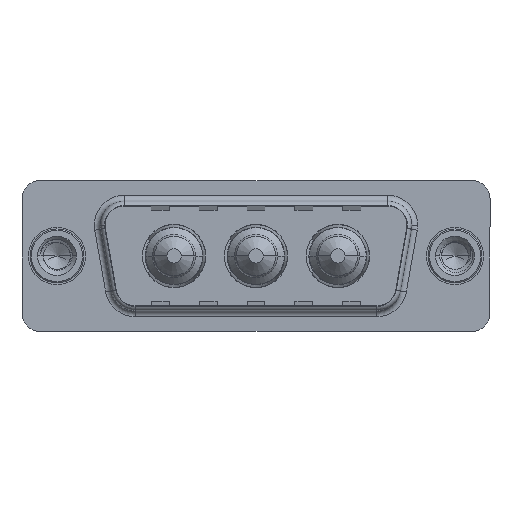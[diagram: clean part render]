
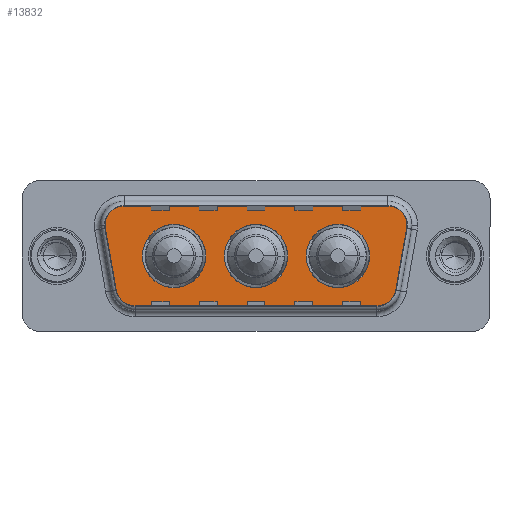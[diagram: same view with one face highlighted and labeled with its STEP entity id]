
A CAD part, top view. The second image highlights one B-rep face of the part: STEP entity #13832.
In plain terms, the highlighted planar face has unit normal (0, 0, 1).
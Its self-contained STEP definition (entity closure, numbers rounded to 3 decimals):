
#61 = DIRECTION ( 'NONE',  ( 0., 0., 1. ) ) ;
#78 = AXIS2_PLACEMENT_3D ( 'NONE', #301, #9163, #1596 ) ;
#163 = EDGE_CURVE ( 'NONE', #9623, #9041, #13083, .T. ) ;
#291 = CIRCLE ( 'NONE', #7058, 2.65 ) ;
#301 = CARTESIAN_POINT ( 'NONE',  ( 6.434, -2.9, 0. ) ) ;
#304 = CARTESIAN_POINT ( 'NONE',  ( 26.866, -2.9, 0. ) ) ;
#387 = EDGE_CURVE ( 'NONE', #11816, #12930, #13210, .T. ) ;
#466 = DIRECTION ( 'NONE',  ( 0., 0., 1. ) ) ;
#569 = VERTEX_POINT ( 'NONE', #11325 ) ;
#781 = EDGE_CURVE ( 'NONE', #16310, #8497, #2176, .T. ) ;
#783 = CIRCLE ( 'NONE', #78, 2. ) ;
#862 = ORIENTED_EDGE ( 'NONE', *, *, #2254, .F. ) ;
#960 = EDGE_LOOP ( 'NONE', ( #14982, #11648 ) ) ;
#1304 = ORIENTED_EDGE ( 'NONE', *, *, #15572, .T. ) ;
#1589 = AXIS2_PLACEMENT_3D ( 'NONE', #7036, #9707, #8698 ) ;
#1596 = DIRECTION ( 'NONE',  ( -1., 0., 0. ) ) ;
#1604 = CIRCLE ( 'NONE', #14845, 2.65 ) ;
#1713 = DIRECTION ( 'NONE',  ( 1., 0., 0. ) ) ;
#2176 = CIRCLE ( 'NONE', #6014, 2. ) ;
#2254 = EDGE_CURVE ( 'NONE', #11732, #569, #14954, .T. ) ;
#2324 = CIRCLE ( 'NONE', #15003, 2. ) ;
#2423 = EDGE_CURVE ( 'NONE', #12930, #9623, #12947, .T. ) ;
#2618 = DIRECTION ( 'NONE',  ( 1., 0., 0. ) ) ;
#2625 = CARTESIAN_POINT ( 'NONE',  ( 29.859, 2.553, 0. ) ) ;
#2858 = CARTESIAN_POINT ( 'NONE',  ( 5.411, 4.9, 0. ) ) ;
#2860 = EDGE_CURVE ( 'NONE', #15848, #16310, #4694, .T. ) ;
#2887 = EDGE_CURVE ( 'NONE', #12675, #8812, #14366, .T. ) ;
#2980 = DIRECTION ( 'NONE',  ( 0., 0., 1. ) ) ;
#3108 = ORIENTED_EDGE ( 'NONE', *, *, #163, .T. ) ;
#3257 = EDGE_CURVE ( 'NONE', #569, #11732, #13745, .T. ) ;
#3400 = CARTESIAN_POINT ( 'NONE',  ( 9.8, 0., 0. ) ) ;
#3410 = CARTESIAN_POINT ( 'NONE',  ( 3.441, 2.553, 0. ) ) ;
#3514 = AXIS2_PLACEMENT_3D ( 'NONE', #6368, #4730, #14247 ) ;
#3944 = ORIENTED_EDGE ( 'NONE', *, *, #781, .T. ) ;
#3976 = DIRECTION ( 'NONE',  ( 1., 0., 0. ) ) ;
#4053 = EDGE_CURVE ( 'NONE', #8812, #12675, #10983, .T. ) ;
#4225 = DIRECTION ( 'NONE',  ( -1., 0., 0. ) ) ;
#4395 = CARTESIAN_POINT ( 'NONE',  ( 3.441, 2.553, 0. ) ) ;
#4661 = DIRECTION ( 'NONE',  ( 1., 0., 0. ) ) ;
#4681 = ORIENTED_EDGE ( 'NONE', *, *, #2887, .F. ) ;
#4694 = LINE ( 'NONE', #5410, #11018 ) ;
#4699 = CARTESIAN_POINT ( 'NONE',  ( 26.866, -2.9, 0. ) ) ;
#4730 = DIRECTION ( 'NONE',  ( 0., 0., 1. ) ) ;
#4750 = CARTESIAN_POINT ( 'NONE',  ( 14., 0., 0. ) ) ;
#4872 = ORIENTED_EDGE ( 'NONE', *, *, #9179, .T. ) ;
#4978 = FACE_OUTER_BOUND ( 'NONE', #7651, .T. ) ;
#5063 = DIRECTION ( 'NONE',  ( -1., 0., 0. ) ) ;
#5396 = DIRECTION ( 'NONE',  ( 1., 0., 0. ) ) ;
#5410 = CARTESIAN_POINT ( 'NONE',  ( 6.434, -4.9, 0. ) ) ;
#5851 = CARTESIAN_POINT ( 'NONE',  ( 26.866, -4.9, 0. ) ) ;
#6014 = AXIS2_PLACEMENT_3D ( 'NONE', #4699, #9716, #1713 ) ;
#6122 = DIRECTION ( 'NONE',  ( 0.174, 0.985, 0. ) ) ;
#6132 = EDGE_CURVE ( 'NONE', #15723, #11286, #1604, .T. ) ;
#6368 = CARTESIAN_POINT ( 'NONE',  ( 23.5, 0., 0. ) ) ;
#6400 = CARTESIAN_POINT ( 'NONE',  ( 23.5, 0., 0. ) ) ;
#6404 = CARTESIAN_POINT ( 'NONE',  ( 27.889, 4.9, 0. ) ) ;
#6472 = CARTESIAN_POINT ( 'NONE',  ( 27.889, 2.9, 0. ) ) ;
#7036 = CARTESIAN_POINT ( 'NONE',  ( 5.411, 2.9, 0. ) ) ;
#7058 = AXIS2_PLACEMENT_3D ( 'NONE', #8048, #466, #9312 ) ;
#7291 = EDGE_LOOP ( 'NONE', ( #11979, #4681 ) ) ;
#7331 = AXIS2_PLACEMENT_3D ( 'NONE', #6400, #61, #2618 ) ;
#7557 = FACE_BOUND ( 'NONE', #7291, .T. ) ;
#7565 = CARTESIAN_POINT ( 'NONE',  ( 5.411, 4.9, 0. ) ) ;
#7587 = CARTESIAN_POINT ( 'NONE',  ( 6.434, -4.9, 0. ) ) ;
#7651 = EDGE_LOOP ( 'NONE', ( #3944, #4872, #14898, #15714, #13138, #3108, #11082, #1304, #13978 ) ) ;
#7766 = DIRECTION ( 'NONE',  ( -1., 0., 0. ) ) ;
#8017 = AXIS2_PLACEMENT_3D ( 'NONE', #304, #12959, #5396 ) ;
#8048 = CARTESIAN_POINT ( 'NONE',  ( 9.8, 0., 0. ) ) ;
#8497 = VERTEX_POINT ( 'NONE', #10308 ) ;
#8698 = DIRECTION ( 'NONE',  ( 1., 0., 0. ) ) ;
#8812 = VERTEX_POINT ( 'NONE', #12828 ) ;
#9041 = VERTEX_POINT ( 'NONE', #3410 ) ;
#9163 = DIRECTION ( 'NONE',  ( 0., 0., 1. ) ) ;
#9179 = EDGE_CURVE ( 'NONE', #8497, #12902, #10656, .T. ) ;
#9204 = VECTOR ( 'NONE', #5063, 1000. ) ;
#9312 = DIRECTION ( 'NONE',  ( 1., 0., 0. ) ) ;
#9623 = VERTEX_POINT ( 'NONE', #2858 ) ;
#9707 = DIRECTION ( 'NONE',  ( 0., 0., 1. ) ) ;
#9716 = DIRECTION ( 'NONE',  ( 0., 0., 1. ) ) ;
#9951 = EDGE_LOOP ( 'NONE', ( #15426, #862 ) ) ;
#10010 = CARTESIAN_POINT ( 'NONE',  ( 29.889, 2.9, 0. ) ) ;
#10082 = CARTESIAN_POINT ( 'NONE',  ( 12.45, 0., 0. ) ) ;
#10250 = DIRECTION ( 'NONE',  ( 1., 0., 0. ) ) ;
#10308 = CARTESIAN_POINT ( 'NONE',  ( 28.836, -3.247, 0. ) ) ;
#10428 = PLANE ( 'NONE',  #8017 ) ;
#10656 = LINE ( 'NONE', #16272, #13998 ) ;
#10679 = VECTOR ( 'NONE', #13199, 1000. ) ;
#10929 = FACE_BOUND ( 'NONE', #9951, .T. ) ;
#10983 = CIRCLE ( 'NONE', #15707, 2.65 ) ;
#11018 = VECTOR ( 'NONE', #10250, 1000. ) ;
#11082 = ORIENTED_EDGE ( 'NONE', *, *, #15251, .T. ) ;
#11087 = LINE ( 'NONE', #4395, #10679 ) ;
#11286 = VERTEX_POINT ( 'NONE', #10082 ) ;
#11325 = CARTESIAN_POINT ( 'NONE',  ( 26.15, 0., 0. ) ) ;
#11386 = DIRECTION ( 'NONE',  ( 0., 0., 1. ) ) ;
#11648 = ORIENTED_EDGE ( 'NONE', *, *, #6132, .F. ) ;
#11732 = VERTEX_POINT ( 'NONE', #13401 ) ;
#11816 = VERTEX_POINT ( 'NONE', #10010 ) ;
#11872 = EDGE_CURVE ( 'NONE', #12902, #11816, #2324, .T. ) ;
#11979 = ORIENTED_EDGE ( 'NONE', *, *, #4053, .F. ) ;
#12032 = EDGE_CURVE ( 'NONE', #11286, #15723, #291, .T. ) ;
#12219 = DIRECTION ( 'NONE',  ( 0., 0., 1. ) ) ;
#12675 = VERTEX_POINT ( 'NONE', #4750 ) ;
#12828 = CARTESIAN_POINT ( 'NONE',  ( 19.3, 0., 0. ) ) ;
#12902 = VERTEX_POINT ( 'NONE', #2625 ) ;
#12930 = VERTEX_POINT ( 'NONE', #6404 ) ;
#12947 = LINE ( 'NONE', #7565, #9204 ) ;
#12959 = DIRECTION ( 'NONE',  ( 0., 0., 1. ) ) ;
#13016 = AXIS2_PLACEMENT_3D ( 'NONE', #13059, #2980, #3976 ) ;
#13059 = CARTESIAN_POINT ( 'NONE',  ( 16.65, 0., 0. ) ) ;
#13083 = CIRCLE ( 'NONE', #1589, 2. ) ;
#13138 = ORIENTED_EDGE ( 'NONE', *, *, #2423, .T. ) ;
#13199 = DIRECTION ( 'NONE',  ( 0.174, -0.985, 0. ) ) ;
#13210 = CIRCLE ( 'NONE', #16015, 2. ) ;
#13278 = DIRECTION ( 'NONE',  ( 0., 0., 1. ) ) ;
#13375 = VERTEX_POINT ( 'NONE', #14599 ) ;
#13401 = CARTESIAN_POINT ( 'NONE',  ( 20.85, 0., 0. ) ) ;
#13699 = CARTESIAN_POINT ( 'NONE',  ( 16.65, 0., 0. ) ) ;
#13745 = CIRCLE ( 'NONE', #7331, 2.65 ) ;
#13832 = ADVANCED_FACE ( 'NONE', ( #7557, #10929, #13861, #4978 ), #10428, .T. ) ;
#13861 = FACE_BOUND ( 'NONE', #960, .T. ) ;
#13978 = ORIENTED_EDGE ( 'NONE', *, *, #2860, .T. ) ;
#13998 = VECTOR ( 'NONE', #6122, 1000. ) ;
#14247 = DIRECTION ( 'NONE',  ( 1., 0., 0. ) ) ;
#14366 = CIRCLE ( 'NONE', #13016, 2.65 ) ;
#14404 = CARTESIAN_POINT ( 'NONE',  ( 27.889, 2.9, 0. ) ) ;
#14599 = CARTESIAN_POINT ( 'NONE',  ( 4.464, -3.247, 0. ) ) ;
#14845 = AXIS2_PLACEMENT_3D ( 'NONE', #3400, #12219, #4661 ) ;
#14898 = ORIENTED_EDGE ( 'NONE', *, *, #11872, .T. ) ;
#14954 = CIRCLE ( 'NONE', #3514, 2.65 ) ;
#14982 = ORIENTED_EDGE ( 'NONE', *, *, #12032, .F. ) ;
#15003 = AXIS2_PLACEMENT_3D ( 'NONE', #6472, #15335, #7766 ) ;
#15251 = EDGE_CURVE ( 'NONE', #9041, #13375, #11087, .T. ) ;
#15335 = DIRECTION ( 'NONE',  ( 0., 0., 1. ) ) ;
#15426 = ORIENTED_EDGE ( 'NONE', *, *, #3257, .F. ) ;
#15572 = EDGE_CURVE ( 'NONE', #13375, #15848, #783, .T. ) ;
#15707 = AXIS2_PLACEMENT_3D ( 'NONE', #13699, #13278, #15776 ) ;
#15714 = ORIENTED_EDGE ( 'NONE', *, *, #387, .T. ) ;
#15723 = VERTEX_POINT ( 'NONE', #15861 ) ;
#15776 = DIRECTION ( 'NONE',  ( 1., 0., 0. ) ) ;
#15848 = VERTEX_POINT ( 'NONE', #7587 ) ;
#15861 = CARTESIAN_POINT ( 'NONE',  ( 7.15, 0., 0. ) ) ;
#16015 = AXIS2_PLACEMENT_3D ( 'NONE', #14404, #11386, #4225 ) ;
#16272 = CARTESIAN_POINT ( 'NONE',  ( 29.859, 2.553, 0. ) ) ;
#16310 = VERTEX_POINT ( 'NONE', #5851 ) ;
